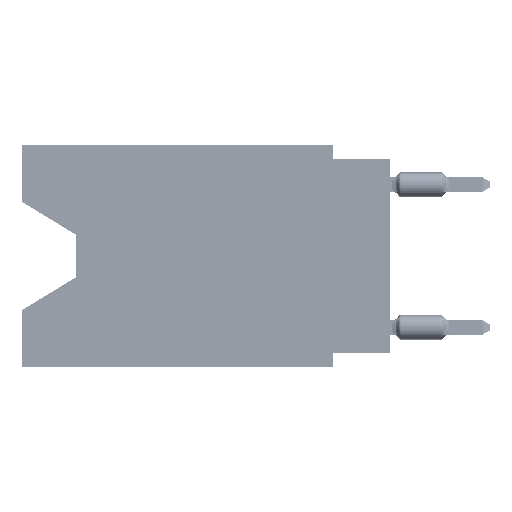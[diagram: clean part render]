
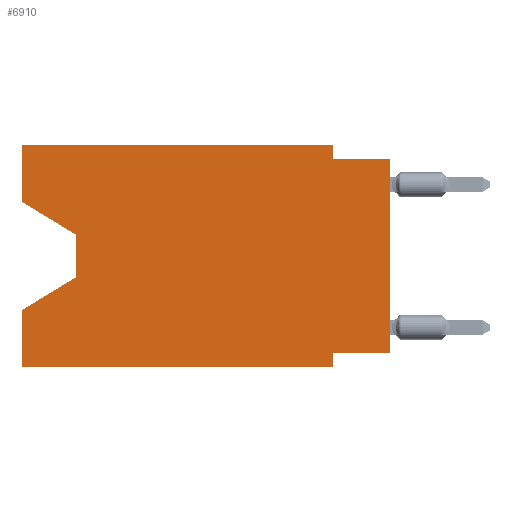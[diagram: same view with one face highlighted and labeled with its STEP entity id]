
A CAD part, left-side view. The second image highlights one B-rep face of the part: STEP entity #6910.
In plain terms, the highlighted planar face has unit normal (-1, 0, 0).
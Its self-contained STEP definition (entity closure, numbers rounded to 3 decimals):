
#311 = DIRECTION ( 'NONE',  ( 0., -1., 0. ) ) ;
#1048 = DIRECTION ( 'NONE',  ( 0., 1., 0. ) ) ;
#3800 = CARTESIAN_POINT ( 'NONE',  ( 0., 2.54, -9.906 ) ) ;
#4124 = VECTOR ( 'NONE', #40999, 1000. ) ;
#5334 = VERTEX_POINT ( 'NONE', #53705 ) ;
#5700 = CARTESIAN_POINT ( 'NONE',  ( 0., 13.97, -5.893 ) ) ;
#6079 = LINE ( 'NONE', #37634, #18166 ) ;
#6413 = PLANE ( 'NONE',  #79296 ) ;
#6565 = VECTOR ( 'NONE', #40136, 1000. ) ;
#6910 = ADVANCED_FACE ( 'NONE', ( #12308 ), #6413, .F. ) ;
#8891 = CARTESIAN_POINT ( 'NONE',  ( 0., 16.383, -9.906 ) ) ;
#9083 = CARTESIAN_POINT ( 'NONE',  ( 0., 16.383, -9.906 ) ) ;
#9337 = ORIENTED_EDGE ( 'NONE', *, *, #49254, .F. ) ;
#11943 = CARTESIAN_POINT ( 'NONE',  ( 0., 16.383, 0. ) ) ;
#12308 = FACE_OUTER_BOUND ( 'NONE', #78459, .T. ) ;
#14370 = ORIENTED_EDGE ( 'NONE', *, *, #73106, .T. ) ;
#15724 = VERTEX_POINT ( 'NONE', #31367 ) ;
#18166 = VECTOR ( 'NONE', #18281, 1000. ) ;
#18265 = EDGE_CURVE ( 'NONE', #20401, #43589, #21701, .T. ) ;
#18281 = DIRECTION ( 'NONE',  ( 0., -0.855, -0.519 ) ) ;
#18605 = DIRECTION ( 'NONE',  ( 0., 0., -1. ) ) ;
#18928 = DIRECTION ( 'NONE',  ( 0., 0., 1. ) ) ;
#19385 = CARTESIAN_POINT ( 'NONE',  ( 0., 0., -0.635 ) ) ;
#19935 = CARTESIAN_POINT ( 'NONE',  ( 0., 0., -9.271 ) ) ;
#20222 = LINE ( 'NONE', #76975, #68317 ) ;
#20401 = VERTEX_POINT ( 'NONE', #8891 ) ;
#20884 = LINE ( 'NONE', #68972, #57756 ) ;
#21701 = LINE ( 'NONE', #9083, #42337 ) ;
#21769 = CARTESIAN_POINT ( 'NONE',  ( 0., 2.54, -9.271 ) ) ;
#22368 = VECTOR ( 'NONE', #50668, 1000. ) ;
#22429 = CARTESIAN_POINT ( 'NONE',  ( 0., 2.54, 0. ) ) ;
#22522 = CARTESIAN_POINT ( 'NONE',  ( 0., 13.97, -4.013 ) ) ;
#23560 = VECTOR ( 'NONE', #1048, 1000. ) ;
#23954 = EDGE_CURVE ( 'NONE', #5334, #37680, #77517, .T. ) ;
#24136 = CARTESIAN_POINT ( 'NONE',  ( 0., 16.383, 0. ) ) ;
#24914 = DIRECTION ( 'NONE',  ( 0., 0., -1. ) ) ;
#25326 = DIRECTION ( 'NONE',  ( 1., 0., 0. ) ) ;
#27943 = CARTESIAN_POINT ( 'NONE',  ( 0., 0., -0.635 ) ) ;
#29747 = VERTEX_POINT ( 'NONE', #32848 ) ;
#29795 = EDGE_CURVE ( 'NONE', #37680, #43589, #20222, .T. ) ;
#30424 = CARTESIAN_POINT ( 'NONE',  ( 0., 16.383, 0. ) ) ;
#30568 = ORIENTED_EDGE ( 'NONE', *, *, #58418, .F. ) ;
#31353 = DIRECTION ( 'NONE',  ( 0., 0.855, -0.519 ) ) ;
#31367 = CARTESIAN_POINT ( 'NONE',  ( 0., 2.54, -0.635 ) ) ;
#31466 = VERTEX_POINT ( 'NONE', #73069 ) ;
#32848 = CARTESIAN_POINT ( 'NONE',  ( 0., 16.383, -7.36 ) ) ;
#33535 = ORIENTED_EDGE ( 'NONE', *, *, #76149, .F. ) ;
#33916 = DIRECTION ( 'NONE',  ( 0., -1., 0. ) ) ;
#34678 = ORIENTED_EDGE ( 'NONE', *, *, #66786, .F. ) ;
#35324 = CARTESIAN_POINT ( 'NONE',  ( 0., 13.97, -5.893 ) ) ;
#37580 = LINE ( 'NONE', #24136, #78068 ) ;
#37634 = CARTESIAN_POINT ( 'NONE',  ( 0., 16.383, -2.546 ) ) ;
#37680 = VERTEX_POINT ( 'NONE', #21769 ) ;
#38261 = VERTEX_POINT ( 'NONE', #11943 ) ;
#38413 = VECTOR ( 'NONE', #24914, 1000. ) ;
#39171 = EDGE_CURVE ( 'NONE', #77599, #41089, #61180, .T. ) ;
#39968 = VERTEX_POINT ( 'NONE', #19385 ) ;
#40136 = DIRECTION ( 'NONE',  ( 0., -1., 0. ) ) ;
#40896 = VECTOR ( 'NONE', #311, 1000. ) ;
#40999 = DIRECTION ( 'NONE',  ( 0., 0., -1. ) ) ;
#41089 = VERTEX_POINT ( 'NONE', #35324 ) ;
#42337 = VECTOR ( 'NONE', #33916, 1000. ) ;
#43589 = VERTEX_POINT ( 'NONE', #3800 ) ;
#45196 = LINE ( 'NONE', #27943, #6565 ) ;
#47987 = ORIENTED_EDGE ( 'NONE', *, *, #59086, .F. ) ;
#49254 = EDGE_CURVE ( 'NONE', #15724, #39968, #45196, .T. ) ;
#50211 = CARTESIAN_POINT ( 'NONE',  ( 0., 13.97, -4.013 ) ) ;
#50668 = DIRECTION ( 'NONE',  ( 0., 0., 1. ) ) ;
#51569 = CARTESIAN_POINT ( 'NONE',  ( 0., 16.383, 0. ) ) ;
#51756 = DIRECTION ( 'NONE',  ( 0., 0., -1. ) ) ;
#51954 = ORIENTED_EDGE ( 'NONE', *, *, #29795, .F. ) ;
#53705 = CARTESIAN_POINT ( 'NONE',  ( 0., 0., -9.271 ) ) ;
#57756 = VECTOR ( 'NONE', #18928, 1000. ) ;
#57846 = ORIENTED_EDGE ( 'NONE', *, *, #18265, .T. ) ;
#58418 = EDGE_CURVE ( 'NONE', #38261, #70357, #70495, .T. ) ;
#59086 = EDGE_CURVE ( 'NONE', #70357, #15724, #74539, .T. ) ;
#61180 = LINE ( 'NONE', #22522, #4124 ) ;
#63284 = CARTESIAN_POINT ( 'NONE',  ( 0., 16.383, 0. ) ) ;
#63294 = LINE ( 'NONE', #5700, #79287 ) ;
#64093 = LINE ( 'NONE', #63284, #22368 ) ;
#65489 = ORIENTED_EDGE ( 'NONE', *, *, #23954, .F. ) ;
#66786 = EDGE_CURVE ( 'NONE', #20401, #29747, #64093, .T. ) ;
#68317 = VECTOR ( 'NONE', #51756, 1000. ) ;
#68972 = CARTESIAN_POINT ( 'NONE',  ( 0., 0., 0. ) ) ;
#69070 = ORIENTED_EDGE ( 'NONE', *, *, #39171, .T. ) ;
#70357 = VERTEX_POINT ( 'NONE', #22429 ) ;
#70495 = LINE ( 'NONE', #51569, #40896 ) ;
#71781 = ORIENTED_EDGE ( 'NONE', *, *, #80614, .T. ) ;
#73069 = CARTESIAN_POINT ( 'NONE',  ( 0., 16.383, -2.546 ) ) ;
#73106 = EDGE_CURVE ( 'NONE', #41089, #29747, #63294, .T. ) ;
#74366 = EDGE_CURVE ( 'NONE', #5334, #39968, #20884, .T. ) ;
#74539 = LINE ( 'NONE', #76195, #38413 ) ;
#75404 = DIRECTION ( 'NONE',  ( 0., 0., 1. ) ) ;
#76149 = EDGE_CURVE ( 'NONE', #31466, #38261, #37580, .T. ) ;
#76195 = CARTESIAN_POINT ( 'NONE',  ( 0., 2.54, 0. ) ) ;
#76975 = CARTESIAN_POINT ( 'NONE',  ( 0., 2.54, -9.906 ) ) ;
#77517 = LINE ( 'NONE', #19935, #23560 ) ;
#77599 = VERTEX_POINT ( 'NONE', #50211 ) ;
#77666 = ORIENTED_EDGE ( 'NONE', *, *, #74366, .T. ) ;
#78068 = VECTOR ( 'NONE', #75404, 1000. ) ;
#78459 = EDGE_LOOP ( 'NONE', ( #71781, #69070, #14370, #34678, #57846, #51954, #65489, #77666, #9337, #47987, #30568, #33535 ) ) ;
#79287 = VECTOR ( 'NONE', #31353, 1000. ) ;
#79296 = AXIS2_PLACEMENT_3D ( 'NONE', #30424, #25326, #18605 ) ;
#80614 = EDGE_CURVE ( 'NONE', #31466, #77599, #6079, .T. ) ;
